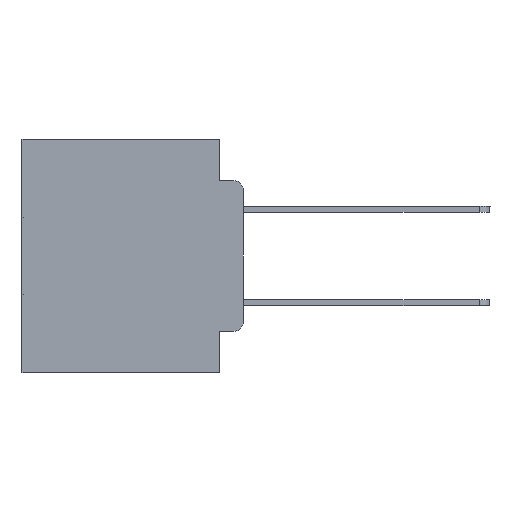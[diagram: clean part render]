
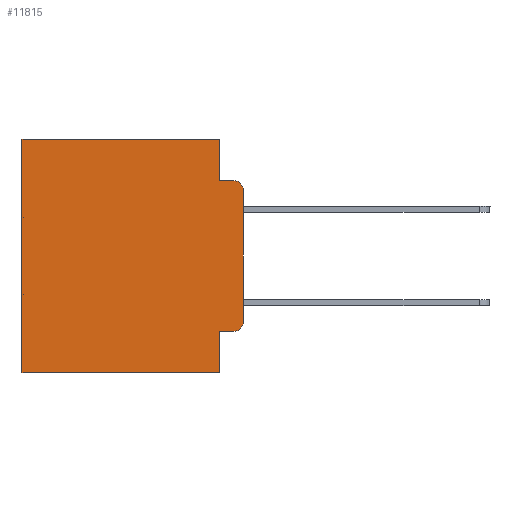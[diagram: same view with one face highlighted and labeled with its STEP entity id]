
A CAD part, left-side view. The second image highlights one B-rep face of the part: STEP entity #11815.
In plain terms, the highlighted planar face has unit normal (-1, 0, 0).
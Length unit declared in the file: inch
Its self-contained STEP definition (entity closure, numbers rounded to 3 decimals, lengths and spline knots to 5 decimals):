
#373 = VERTEX_POINT ( 'NONE', #10760 ) ;
#963 = AXIS2_PLACEMENT_3D ( 'NONE', #1409, #6340, #23240 ) ;
#1409 = CARTESIAN_POINT ( 'NONE',  ( 0.298, 0., 0. ) ) ;
#1462 = ORIENTED_EDGE ( 'NONE', *, *, #17778, .T. ) ;
#1791 = CIRCLE ( 'NONE', #28817, 0.02 ) ;
#1905 = DIRECTION ( 'NONE',  ( 0., 0., -1. ) ) ;
#1985 = VERTEX_POINT ( 'NONE', #17677 ) ;
#2137 = CARTESIAN_POINT ( 'NONE',  ( 0.298, 0., -0.1085 ) ) ;
#2180 = FACE_OUTER_BOUND ( 'NONE', #23736, .T. ) ;
#3113 = VECTOR ( 'NONE', #27500, 39.37008 ) ;
#3372 = VERTEX_POINT ( 'NONE', #19231 ) ;
#3463 = VERTEX_POINT ( 'NONE', #10155 ) ;
#3525 = EDGE_CURVE ( 'NONE', #1985, #3463, #10891, .T. ) ;
#3890 = PLANE ( 'NONE',  #963 ) ;
#4433 = VECTOR ( 'NONE', #18845, 39.37008 ) ;
#5162 = LINE ( 'NONE', #29784, #23688 ) ;
#5309 = DIRECTION ( 'NONE',  ( 0., -1., 0. ) ) ;
#5654 = CARTESIAN_POINT ( 'NONE',  ( 0.298, 0.02, -0.0885 ) ) ;
#5900 = CARTESIAN_POINT ( 'NONE',  ( 0.298, 0.051, -0.0885 ) ) ;
#5998 = CARTESIAN_POINT ( 'NONE',  ( 0.298, 0.02, -0.3915 ) ) ;
#6085 = LINE ( 'NONE', #16958, #30873 ) ;
#6340 = DIRECTION ( 'NONE',  ( 1., 0., 0. ) ) ;
#6841 = ORIENTED_EDGE ( 'NONE', *, *, #15849, .F. ) ;
#7556 = CARTESIAN_POINT ( 'NONE',  ( 0.298, 0.051, 0. ) ) ;
#8177 = DIRECTION ( 'NONE',  ( 0., 0., -1. ) ) ;
#8423 = VECTOR ( 'NONE', #18009, 39.37008 ) ;
#8461 = DIRECTION ( 'NONE',  ( 0., 0., -1. ) ) ;
#8733 = ORIENTED_EDGE ( 'NONE', *, *, #31198, .F. ) ;
#9128 = VERTEX_POINT ( 'NONE', #27159 ) ;
#9614 = LINE ( 'NONE', #5900, #3113 ) ;
#9821 = DIRECTION ( 'NONE',  ( 0., 0., -1. ) ) ;
#10155 = CARTESIAN_POINT ( 'NONE',  ( 0.298, 0.473, 0. ) ) ;
#10433 = CIRCLE ( 'NONE', #31255, 0.02 ) ;
#10728 = VERTEX_POINT ( 'NONE', #2137 ) ;
#10760 = CARTESIAN_POINT ( 'NONE',  ( 0.298, 0.051, -0.0885 ) ) ;
#10891 = LINE ( 'NONE', #19095, #4433 ) ;
#11815 = ADVANCED_FACE ( 'NONE', ( #2180 ), #3890, .F. ) ;
#12402 = CARTESIAN_POINT ( 'NONE',  ( 0.298, 0.051, -0.4115 ) ) ;
#13504 = EDGE_CURVE ( 'NONE', #3463, #9128, #5162, .T. ) ;
#13967 = EDGE_CURVE ( 'NONE', #21850, #3372, #24385, .T. ) ;
#14828 = ORIENTED_EDGE ( 'NONE', *, *, #25798, .F. ) ;
#14892 = ORIENTED_EDGE ( 'NONE', *, *, #15190, .F. ) ;
#15190 = EDGE_CURVE ( 'NONE', #373, #27833, #9614, .T. ) ;
#15346 = CARTESIAN_POINT ( 'NONE',  ( 0.298, 0.02, -0.4115 ) ) ;
#15556 = ORIENTED_EDGE ( 'NONE', *, *, #13967, .F. ) ;
#15575 = CARTESIAN_POINT ( 'NONE',  ( 0.298, 0., -0.5 ) ) ;
#15849 = EDGE_CURVE ( 'NONE', #3372, #9128, #27603, .T. ) ;
#16444 = DIRECTION ( 'NONE',  ( -1., 0., 0. ) ) ;
#16958 = CARTESIAN_POINT ( 'NONE',  ( 0.298, 0., 0. ) ) ;
#17057 = ORIENTED_EDGE ( 'NONE', *, *, #23639, .T. ) ;
#17677 = CARTESIAN_POINT ( 'NONE',  ( 0.298, 0.051, 0. ) ) ;
#17778 = EDGE_CURVE ( 'NONE', #10728, #27833, #1791, .T. ) ;
#18009 = DIRECTION ( 'NONE',  ( 0., 1., 0. ) ) ;
#18845 = DIRECTION ( 'NONE',  ( 0., 1., 0. ) ) ;
#19095 = CARTESIAN_POINT ( 'NONE',  ( 0.298, 0., 0. ) ) ;
#19231 = CARTESIAN_POINT ( 'NONE',  ( 0.298, 0.051, -0.5 ) ) ;
#20400 = VECTOR ( 'NONE', #22127, 39.37008 ) ;
#21566 = ORIENTED_EDGE ( 'NONE', *, *, #26524, .T. ) ;
#21850 = VERTEX_POINT ( 'NONE', #12402 ) ;
#21960 = CARTESIAN_POINT ( 'NONE',  ( 0.298, 0.051, 0. ) ) ;
#22127 = DIRECTION ( 'NONE',  ( 0., 0., -1. ) ) ;
#22771 = ORIENTED_EDGE ( 'NONE', *, *, #3525, .T. ) ;
#22907 = VECTOR ( 'NONE', #24372, 39.37008 ) ;
#22928 = DIRECTION ( 'NONE',  ( -1., 0., 0. ) ) ;
#23240 = DIRECTION ( 'NONE',  ( 0., 0., -1. ) ) ;
#23639 = EDGE_CURVE ( 'NONE', #24748, #30000, #10433, .T. ) ;
#23688 = VECTOR ( 'NONE', #8177, 39.37008 ) ;
#23736 = EDGE_LOOP ( 'NONE', ( #14828, #1462, #14892, #8733, #22771, #25312, #6841, #15556, #21566, #17057 ) ) ;
#24372 = DIRECTION ( 'NONE',  ( 0., 0., -1. ) ) ;
#24385 = LINE ( 'NONE', #21960, #22907 ) ;
#24748 = VERTEX_POINT ( 'NONE', #15346 ) ;
#24927 = VECTOR ( 'NONE', #5309, 39.37008 ) ;
#25312 = ORIENTED_EDGE ( 'NONE', *, *, #13504, .T. ) ;
#25798 = EDGE_CURVE ( 'NONE', #10728, #30000, #6085, .T. ) ;
#26524 = EDGE_CURVE ( 'NONE', #21850, #24748, #29008, .T. ) ;
#26767 = LINE ( 'NONE', #7556, #20400 ) ;
#26902 = CARTESIAN_POINT ( 'NONE',  ( 0.298, 0.051, -0.4115 ) ) ;
#27159 = CARTESIAN_POINT ( 'NONE',  ( 0.298, 0.473, -0.5 ) ) ;
#27500 = DIRECTION ( 'NONE',  ( 0., -1., 0. ) ) ;
#27603 = LINE ( 'NONE', #15575, #8423 ) ;
#27833 = VERTEX_POINT ( 'NONE', #5654 ) ;
#28817 = AXIS2_PLACEMENT_3D ( 'NONE', #30758, #16444, #1905 ) ;
#29008 = LINE ( 'NONE', #26902, #24927 ) ;
#29571 = CARTESIAN_POINT ( 'NONE',  ( 0.298, 0., -0.3915 ) ) ;
#29784 = CARTESIAN_POINT ( 'NONE',  ( 0.298, 0.473, 0. ) ) ;
#30000 = VERTEX_POINT ( 'NONE', #29571 ) ;
#30758 = CARTESIAN_POINT ( 'NONE',  ( 0.298, 0.02, -0.1085 ) ) ;
#30873 = VECTOR ( 'NONE', #9821, 39.37008 ) ;
#31198 = EDGE_CURVE ( 'NONE', #1985, #373, #26767, .T. ) ;
#31255 = AXIS2_PLACEMENT_3D ( 'NONE', #5998, #22928, #8461 ) ;
